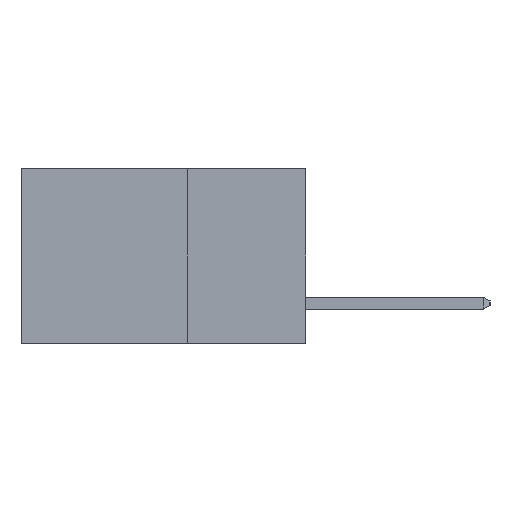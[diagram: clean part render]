
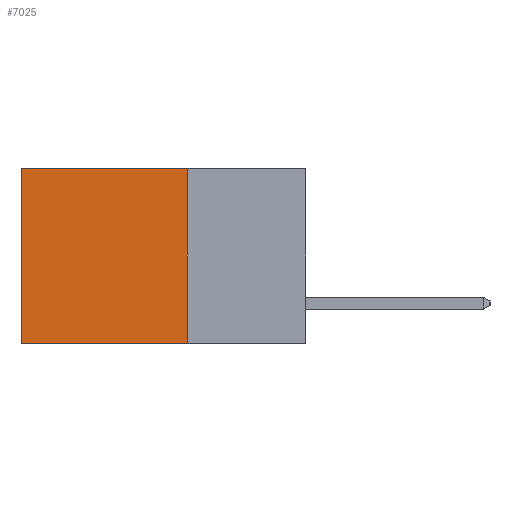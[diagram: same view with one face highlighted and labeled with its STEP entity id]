
A CAD part, left-side view. The second image highlights one B-rep face of the part: STEP entity #7025.
In plain terms, the highlighted planar face has unit normal (-1, 0, 0).
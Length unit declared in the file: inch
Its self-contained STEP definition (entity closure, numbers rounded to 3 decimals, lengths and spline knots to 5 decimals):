
#207 = CARTESIAN_POINT ( 'NONE',  ( 0.298, 0.25, -0.37 ) ) ;
#291 = DIRECTION ( 'NONE',  ( 0., 0., -1. ) ) ;
#351 = DIRECTION ( 'NONE',  ( 0., 0., -1. ) ) ;
#1076 = VECTOR ( 'NONE', #7889, 39.37008 ) ;
#1146 = CARTESIAN_POINT ( 'NONE',  ( 0.298, 0.6, 0. ) ) ;
#1550 = CARTESIAN_POINT ( 'NONE',  ( 0.298, 0.25, 0. ) ) ;
#1602 = VERTEX_POINT ( 'NONE', #1550 ) ;
#2109 = LINE ( 'NONE', #3853, #6888 ) ;
#2301 = LINE ( 'NONE', #7380, #9825 ) ;
#2735 = VERTEX_POINT ( 'NONE', #6207 ) ;
#3736 = EDGE_LOOP ( 'NONE', ( #10304, #6781, #9624, #10837 ) ) ;
#3754 = EDGE_CURVE ( 'NONE', #4291, #2735, #2301, .T. ) ;
#3853 = CARTESIAN_POINT ( 'NONE',  ( 0.298, 0.25, 0. ) ) ;
#4201 = PLANE ( 'NONE',  #10897 ) ;
#4291 = VERTEX_POINT ( 'NONE', #207 ) ;
#4825 = DIRECTION ( 'NONE',  ( 0., 1., 0. ) ) ;
#4895 = EDGE_CURVE ( 'NONE', #1602, #4291, #6193, .T. ) ;
#5115 = CARTESIAN_POINT ( 'NONE',  ( 0.298, 0.6, 0. ) ) ;
#6121 = DIRECTION ( 'NONE',  ( 1., 0., 0. ) ) ;
#6193 = LINE ( 'NONE', #6953, #1076 ) ;
#6207 = CARTESIAN_POINT ( 'NONE',  ( 0.298, 0.6, -0.37 ) ) ;
#6781 = ORIENTED_EDGE ( 'NONE', *, *, #3754, .F. ) ;
#6888 = VECTOR ( 'NONE', #4825, 39.37008 ) ;
#6953 = CARTESIAN_POINT ( 'NONE',  ( 0.298, 0.25, 0. ) ) ;
#7025 = ADVANCED_FACE ( 'NONE', ( #12152 ), #4201, .F. ) ;
#7380 = CARTESIAN_POINT ( 'NONE',  ( 0.298, 0.25, -0.37 ) ) ;
#7484 = EDGE_CURVE ( 'NONE', #1602, #9775, #2109, .T. ) ;
#7889 = DIRECTION ( 'NONE',  ( 0., 0., -1. ) ) ;
#7903 = VECTOR ( 'NONE', #291, 39.37008 ) ;
#9027 = DIRECTION ( 'NONE',  ( 0., 1., 0. ) ) ;
#9624 = ORIENTED_EDGE ( 'NONE', *, *, #4895, .F. ) ;
#9775 = VERTEX_POINT ( 'NONE', #1146 ) ;
#9825 = VECTOR ( 'NONE', #9027, 39.37008 ) ;
#10304 = ORIENTED_EDGE ( 'NONE', *, *, #10461, .T. ) ;
#10339 = LINE ( 'NONE', #5115, #7903 ) ;
#10461 = EDGE_CURVE ( 'NONE', #9775, #2735, #10339, .T. ) ;
#10837 = ORIENTED_EDGE ( 'NONE', *, *, #7484, .T. ) ;
#10897 = AXIS2_PLACEMENT_3D ( 'NONE', #11624, #6121, #351 ) ;
#11624 = CARTESIAN_POINT ( 'NONE',  ( 0.298, 0.25, 0. ) ) ;
#12152 = FACE_OUTER_BOUND ( 'NONE', #3736, .T. ) ;
